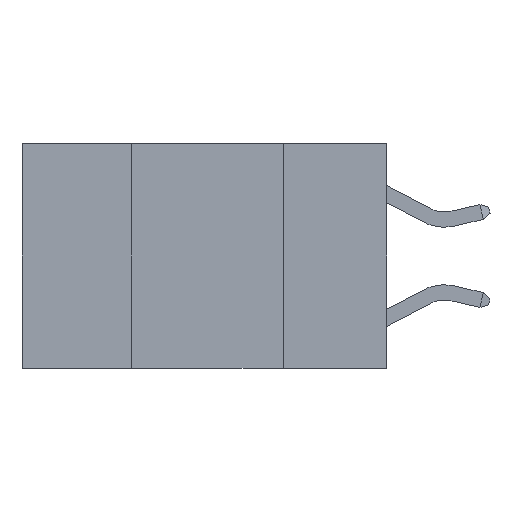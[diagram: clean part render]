
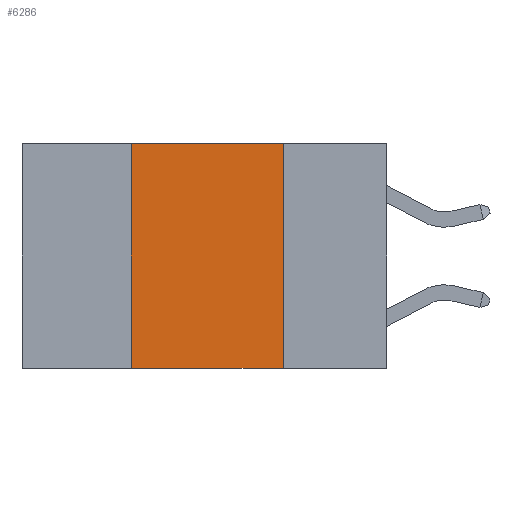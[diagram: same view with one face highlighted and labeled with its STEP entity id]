
A CAD part, left-side view. The second image highlights one B-rep face of the part: STEP entity #6286.
In plain terms, the highlighted planar face has unit normal (-1, 0, 0).
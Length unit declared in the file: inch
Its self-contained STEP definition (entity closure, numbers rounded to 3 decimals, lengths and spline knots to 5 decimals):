
#1 = FACE_OUTER_BOUND ( 'NONE', #600, .T. ) ;
#52 = AXIS2_PLACEMENT_3D ( 'NONE', #8692, #7281, #2730 ) ;
#100 = CARTESIAN_POINT ( 'NONE',  ( 0., 0.42, 0. ) ) ;
#207 = EDGE_CURVE ( 'NONE', #3012, #9511, #8792, .T. ) ;
#416 = ORIENTED_EDGE ( 'NONE', *, *, #750, .F. ) ;
#480 = LINE ( 'NONE', #100, #2093 ) ;
#600 = EDGE_LOOP ( 'NONE', ( #416, #5031, #3246, #6942 ) ) ;
#744 = VECTOR ( 'NONE', #7056, 39.37008 ) ;
#750 = EDGE_CURVE ( 'NONE', #9014, #9511, #7667, .T. ) ;
#976 = CARTESIAN_POINT ( 'NONE',  ( 0., 0.17, 0. ) ) ;
#1773 = DIRECTION ( 'NONE',  ( 0., 0., -1. ) ) ;
#2093 = VECTOR ( 'NONE', #7046, 39.37008 ) ;
#2730 = DIRECTION ( 'NONE',  ( 0., 0., -1. ) ) ;
#2813 = LINE ( 'NONE', #6217, #6634 ) ;
#2973 = CARTESIAN_POINT ( 'NONE',  ( 0., 0.42, 0. ) ) ;
#3012 = VERTEX_POINT ( 'NONE', #5997 ) ;
#3246 = ORIENTED_EDGE ( 'NONE', *, *, #6718, .F. ) ;
#4743 = CARTESIAN_POINT ( 'NONE',  ( 0., 0.17, -0.37 ) ) ;
#5031 = ORIENTED_EDGE ( 'NONE', *, *, #6665, .F. ) ;
#5449 = CARTESIAN_POINT ( 'NONE',  ( 0., 0.17, 0. ) ) ;
#5926 = VECTOR ( 'NONE', #1773, 39.37008 ) ;
#5997 = CARTESIAN_POINT ( 'NONE',  ( 0., 0.42, -0.37 ) ) ;
#6217 = CARTESIAN_POINT ( 'NONE',  ( 0., 0.6, 0. ) ) ;
#6286 = ADVANCED_FACE ( 'NONE', ( #1 ), #6517, .F. ) ;
#6517 = PLANE ( 'NONE',  #52 ) ;
#6634 = VECTOR ( 'NONE', #6982, 39.37008 ) ;
#6665 = EDGE_CURVE ( 'NONE', #7119, #9014, #2813, .T. ) ;
#6718 = EDGE_CURVE ( 'NONE', #3012, #7119, #480, .T. ) ;
#6942 = ORIENTED_EDGE ( 'NONE', *, *, #207, .T. ) ;
#6982 = DIRECTION ( 'NONE',  ( 0., -1., 0. ) ) ;
#7046 = DIRECTION ( 'NONE',  ( 0., 0., 1. ) ) ;
#7056 = DIRECTION ( 'NONE',  ( 0., -1., 0. ) ) ;
#7119 = VERTEX_POINT ( 'NONE', #2973 ) ;
#7281 = DIRECTION ( 'NONE',  ( 1., 0., 0. ) ) ;
#7667 = LINE ( 'NONE', #976, #5926 ) ;
#8584 = CARTESIAN_POINT ( 'NONE',  ( 0., 0.6, -0.37 ) ) ;
#8692 = CARTESIAN_POINT ( 'NONE',  ( 0., 0.6, 0. ) ) ;
#8792 = LINE ( 'NONE', #8584, #744 ) ;
#9014 = VERTEX_POINT ( 'NONE', #5449 ) ;
#9511 = VERTEX_POINT ( 'NONE', #4743 ) ;
